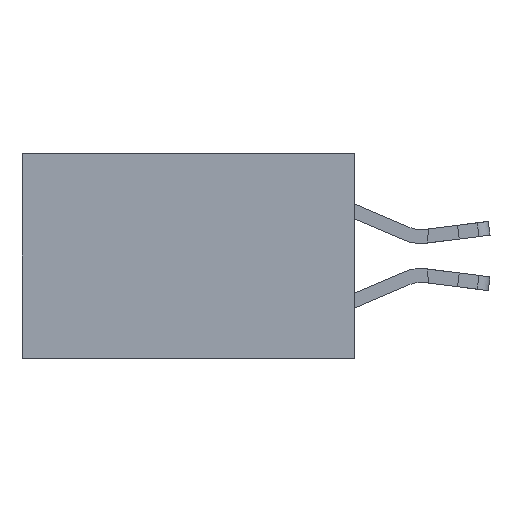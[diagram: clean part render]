
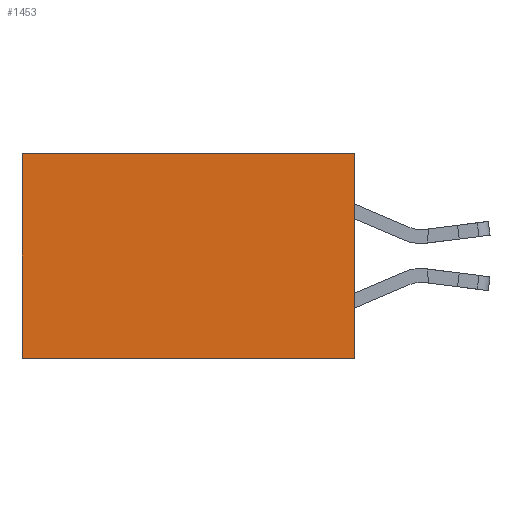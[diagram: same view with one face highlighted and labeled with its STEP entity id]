
A CAD part, left-side view. The second image highlights one B-rep face of the part: STEP entity #1453.
In plain terms, the highlighted planar face has unit normal (-1, 0, 0).
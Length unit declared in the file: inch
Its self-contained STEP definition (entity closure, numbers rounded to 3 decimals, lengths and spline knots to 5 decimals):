
#63 = EDGE_CURVE ( 'NONE', #15988, #20989, #15993, .T. ) ;
#757 = VECTOR ( 'NONE', #16773, 39.37008 ) ;
#887 = DIRECTION ( 'NONE',  ( 0., 0., -1. ) ) ;
#1453 = ADVANCED_FACE ( 'NONE', ( #21056 ), #10271, .F. ) ;
#2128 = ORIENTED_EDGE ( 'NONE', *, *, #8485, .T. ) ;
#2692 = EDGE_CURVE ( 'NONE', #20989, #22665, #19019, .T. ) ;
#3765 = CARTESIAN_POINT ( 'NONE',  ( 0.298, 0.6, 0. ) ) ;
#4085 = DIRECTION ( 'NONE',  ( 0., 0., -1. ) ) ;
#4655 = ORIENTED_EDGE ( 'NONE', *, *, #11280, .T. ) ;
#5003 = AXIS2_PLACEMENT_3D ( 'NONE', #22771, #19250, #4085 ) ;
#5053 = ORIENTED_EDGE ( 'NONE', *, *, #63, .F. ) ;
#5510 = CARTESIAN_POINT ( 'NONE',  ( 0.298, 0., 0. ) ) ;
#6484 = VERTEX_POINT ( 'NONE', #15192 ) ;
#6626 = LINE ( 'NONE', #18809, #11125 ) ;
#7842 = CARTESIAN_POINT ( 'NONE',  ( 0.298, 0., -0.37 ) ) ;
#8485 = EDGE_CURVE ( 'NONE', #6484, #22665, #13811, .T. ) ;
#8874 = VECTOR ( 'NONE', #887, 39.37008 ) ;
#9958 = DIRECTION ( 'NONE',  ( 0., 1., 0. ) ) ;
#10271 = PLANE ( 'NONE',  #5003 ) ;
#10403 = CARTESIAN_POINT ( 'NONE',  ( 0.298, 0., -0.37 ) ) ;
#11125 = VECTOR ( 'NONE', #24027, 39.37008 ) ;
#11280 = EDGE_CURVE ( 'NONE', #15988, #6484, #6626, .T. ) ;
#13811 = LINE ( 'NONE', #3765, #8874 ) ;
#14189 = VECTOR ( 'NONE', #9958, 39.37008 ) ;
#14636 = CARTESIAN_POINT ( 'NONE',  ( 0.298, 0., 0. ) ) ;
#15192 = CARTESIAN_POINT ( 'NONE',  ( 0.298, 0.6, 0. ) ) ;
#15970 = EDGE_LOOP ( 'NONE', ( #2128, #23492, #5053, #4655 ) ) ;
#15988 = VERTEX_POINT ( 'NONE', #14636 ) ;
#15993 = LINE ( 'NONE', #5510, #757 ) ;
#16773 = DIRECTION ( 'NONE',  ( 0., 0., -1. ) ) ;
#18444 = CARTESIAN_POINT ( 'NONE',  ( 0.298, 0.6, -0.37 ) ) ;
#18809 = CARTESIAN_POINT ( 'NONE',  ( 0.298, 0., 0. ) ) ;
#19019 = LINE ( 'NONE', #10403, #14189 ) ;
#19250 = DIRECTION ( 'NONE',  ( 1., 0., 0. ) ) ;
#20989 = VERTEX_POINT ( 'NONE', #7842 ) ;
#21056 = FACE_OUTER_BOUND ( 'NONE', #15970, .T. ) ;
#22665 = VERTEX_POINT ( 'NONE', #18444 ) ;
#22771 = CARTESIAN_POINT ( 'NONE',  ( 0.298, 0., 0. ) ) ;
#23492 = ORIENTED_EDGE ( 'NONE', *, *, #2692, .F. ) ;
#24027 = DIRECTION ( 'NONE',  ( 0., 1., 0. ) ) ;
